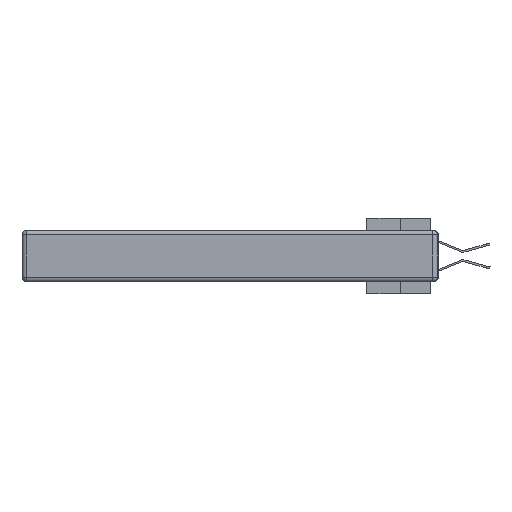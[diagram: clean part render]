
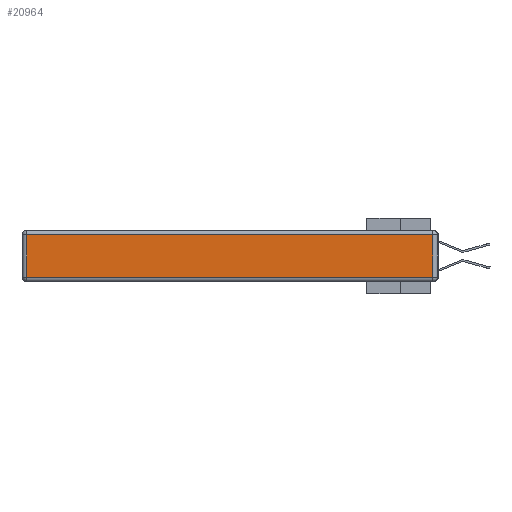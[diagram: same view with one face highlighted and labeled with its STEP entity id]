
A CAD part, left-side view. The second image highlights one B-rep face of the part: STEP entity #20964.
In plain terms, the highlighted planar face has unit normal (-1, 0, 0).
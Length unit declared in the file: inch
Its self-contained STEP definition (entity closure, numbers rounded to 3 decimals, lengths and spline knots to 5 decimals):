
#165 = ORIENTED_EDGE ( 'NONE', *, *, #5946, .T. ) ;
#898 = DIRECTION ( 'NONE',  ( 0., -1., 0. ) ) ;
#1486 = PLANE ( 'NONE',  #32704 ) ;
#1661 = CARTESIAN_POINT ( 'NONE',  ( 0., 2.72, -0.343 ) ) ;
#5946 = EDGE_CURVE ( 'NONE', #8402, #9705, #31603, .T. ) ;
#6915 = DIRECTION ( 'NONE',  ( 0., 0., 1. ) ) ;
#8402 = VERTEX_POINT ( 'NONE', #16020 ) ;
#9435 = CARTESIAN_POINT ( 'NONE',  ( 0., 0.03, -0.343 ) ) ;
#9705 = VERTEX_POINT ( 'NONE', #21940 ) ;
#9865 = DIRECTION ( 'NONE',  ( 0., 0., -1. ) ) ;
#12065 = DIRECTION ( 'NONE',  ( 0., 0., 1. ) ) ;
#12312 = ORIENTED_EDGE ( 'NONE', *, *, #27681, .T. ) ;
#14020 = EDGE_CURVE ( 'NONE', #9705, #25515, #14992, .T. ) ;
#14992 = LINE ( 'NONE', #9435, #19949 ) ;
#15052 = LINE ( 'NONE', #1661, #15463 ) ;
#15463 = VECTOR ( 'NONE', #9865, 39.37008 ) ;
#15695 = EDGE_LOOP ( 'NONE', ( #165, #20404, #12312, #22581 ) ) ;
#16020 = CARTESIAN_POINT ( 'NONE',  ( 0., 2.72, -0.313 ) ) ;
#16389 = CARTESIAN_POINT ( 'NONE',  ( 0., 2.75, -0.03 ) ) ;
#17424 = VECTOR ( 'NONE', #31989, 39.37008 ) ;
#17592 = FACE_OUTER_BOUND ( 'NONE', #15695, .T. ) ;
#19940 = CARTESIAN_POINT ( 'NONE',  ( 0., 0., -0.343 ) ) ;
#19949 = VECTOR ( 'NONE', #12065, 39.37008 ) ;
#20404 = ORIENTED_EDGE ( 'NONE', *, *, #14020, .T. ) ;
#20964 = ADVANCED_FACE ( 'NONE', ( #17592 ), #1486, .T. ) ;
#21589 = EDGE_CURVE ( 'NONE', #32418, #8402, #15052, .T. ) ;
#21940 = CARTESIAN_POINT ( 'NONE',  ( 0., 0.03, -0.313 ) ) ;
#22114 = CARTESIAN_POINT ( 'NONE',  ( 0., 0., -0.313 ) ) ;
#22581 = ORIENTED_EDGE ( 'NONE', *, *, #21589, .T. ) ;
#23411 = VECTOR ( 'NONE', #898, 39.37008 ) ;
#25515 = VERTEX_POINT ( 'NONE', #25573 ) ;
#25573 = CARTESIAN_POINT ( 'NONE',  ( 0., 0.03, -0.03 ) ) ;
#27681 = EDGE_CURVE ( 'NONE', #25515, #32418, #33028, .T. ) ;
#28991 = CARTESIAN_POINT ( 'NONE',  ( 0., 2.72, -0.03 ) ) ;
#31603 = LINE ( 'NONE', #22114, #23411 ) ;
#31989 = DIRECTION ( 'NONE',  ( 0., 1., 0. ) ) ;
#32418 = VERTEX_POINT ( 'NONE', #28991 ) ;
#32704 = AXIS2_PLACEMENT_3D ( 'NONE', #19940, #33486, #6915 ) ;
#33028 = LINE ( 'NONE', #16389, #17424 ) ;
#33486 = DIRECTION ( 'NONE',  ( -1., 0., 0. ) ) ;
